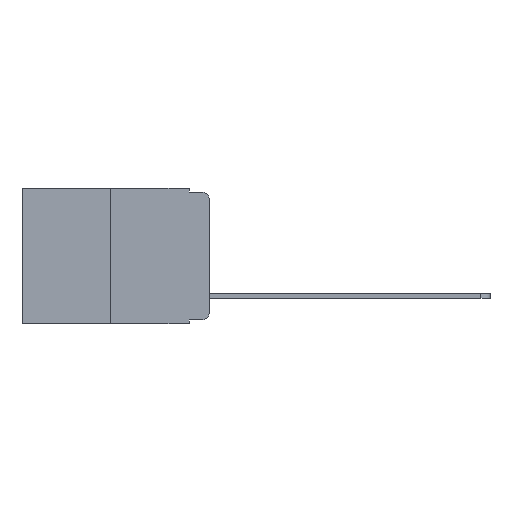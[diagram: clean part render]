
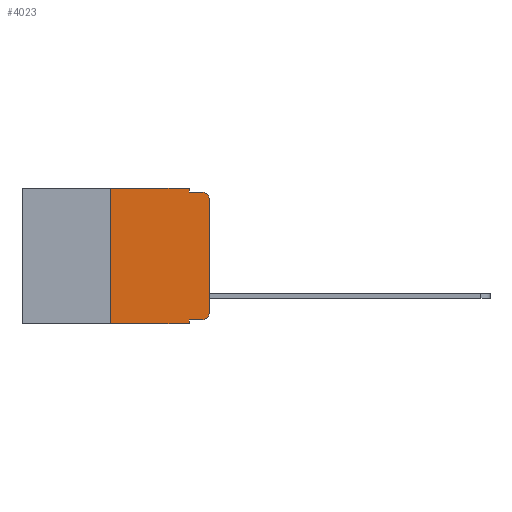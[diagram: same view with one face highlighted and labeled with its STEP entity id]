
A CAD part, left-side view. The second image highlights one B-rep face of the part: STEP entity #4023.
In plain terms, the highlighted planar face has unit normal (-1, 0, 0).
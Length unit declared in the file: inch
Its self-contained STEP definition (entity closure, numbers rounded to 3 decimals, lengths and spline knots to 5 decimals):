
#43 = PLANE ( 'NONE',  #14361 ) ;
#63 = CARTESIAN_POINT ( 'NONE',  ( 0., 0.473, 0. ) ) ;
#77 = CIRCLE ( 'NONE', #10396, 0.02 ) ;
#205 = VECTOR ( 'NONE', #4511, 39.37008 ) ;
#252 = DIRECTION ( 'NONE',  ( 1., 0., 0. ) ) ;
#527 = CARTESIAN_POINT ( 'NONE',  ( 0., 0.25, -0.343 ) ) ;
#549 = LINE ( 'NONE', #7232, #3117 ) ;
#1251 = CARTESIAN_POINT ( 'NONE',  ( 0., 0.051, -0.343 ) ) ;
#1499 = VECTOR ( 'NONE', #2564, 39.37008 ) ;
#1754 = AXIS2_PLACEMENT_3D ( 'NONE', #3244, #12026, #4750 ) ;
#2564 = DIRECTION ( 'NONE',  ( 0., -1., 0. ) ) ;
#2628 = EDGE_LOOP ( 'NONE', ( #7065, #13607, #7468, #11190, #14346, #11562, #14711, #11953, #15067, #15421 ) ) ;
#2665 = CARTESIAN_POINT ( 'NONE',  ( 0., 0.051, -0.333 ) ) ;
#3117 = VECTOR ( 'NONE', #8499, 39.37008 ) ;
#3171 = DIRECTION ( 'NONE',  ( -1., 0., 0. ) ) ;
#3209 = VECTOR ( 'NONE', #5372, 39.37008 ) ;
#3244 = CARTESIAN_POINT ( 'NONE',  ( 0., 0.02, -0.03 ) ) ;
#4023 = ADVANCED_FACE ( 'NONE', ( #10463 ), #43, .F. ) ;
#4182 = DIRECTION ( 'NONE',  ( 0., -1., 0. ) ) ;
#4190 = VECTOR ( 'NONE', #10256, 39.37008 ) ;
#4368 = DIRECTION ( 'NONE',  ( 0., 0., -1. ) ) ;
#4511 = DIRECTION ( 'NONE',  ( 0., 0., 1. ) ) ;
#4624 = VECTOR ( 'NONE', #4182, 39.37008 ) ;
#4635 = LINE ( 'NONE', #13054, #10944 ) ;
#4750 = DIRECTION ( 'NONE',  ( 0., 0., -1. ) ) ;
#5372 = DIRECTION ( 'NONE',  ( 0., 0., -1. ) ) ;
#5976 = EDGE_CURVE ( 'NONE', #7205, #10261, #10786, .T. ) ;
#6073 = CARTESIAN_POINT ( 'NONE',  ( 0., 0.02, -0.01 ) ) ;
#6177 = CARTESIAN_POINT ( 'NONE',  ( 0., 0.02, -0.333 ) ) ;
#6295 = EDGE_CURVE ( 'NONE', #7839, #15605, #77, .T. ) ;
#6835 = CIRCLE ( 'NONE', #1754, 0.02 ) ;
#6948 = LINE ( 'NONE', #7053, #205 ) ;
#7053 = CARTESIAN_POINT ( 'NONE',  ( 0., 0.25, 0. ) ) ;
#7065 = ORIENTED_EDGE ( 'NONE', *, *, #11036, .T. ) ;
#7174 = VECTOR ( 'NONE', #14970, 39.37008 ) ;
#7205 = VERTEX_POINT ( 'NONE', #10015 ) ;
#7232 = CARTESIAN_POINT ( 'NONE',  ( 0., 0.473, -0.343 ) ) ;
#7468 = ORIENTED_EDGE ( 'NONE', *, *, #5976, .F. ) ;
#7551 = LINE ( 'NONE', #2665, #4190 ) ;
#7697 = CARTESIAN_POINT ( 'NONE',  ( 0., 0., 0. ) ) ;
#7839 = VERTEX_POINT ( 'NONE', #6177 ) ;
#7983 = EDGE_CURVE ( 'NONE', #9627, #7839, #7551, .T. ) ;
#8139 = CARTESIAN_POINT ( 'NONE',  ( 0., 0., -0.313 ) ) ;
#8172 = VERTEX_POINT ( 'NONE', #11847 ) ;
#8423 = EDGE_CURVE ( 'NONE', #8839, #10991, #549, .T. ) ;
#8499 = DIRECTION ( 'NONE',  ( 0., -1., 0. ) ) ;
#8839 = VERTEX_POINT ( 'NONE', #527 ) ;
#9021 = DIRECTION ( 'NONE',  ( 0., 0., -1. ) ) ;
#9627 = VERTEX_POINT ( 'NONE', #15664 ) ;
#10015 = CARTESIAN_POINT ( 'NONE',  ( 0., 0.051, -0.01 ) ) ;
#10222 = EDGE_CURVE ( 'NONE', #13345, #10261, #6835, .T. ) ;
#10256 = DIRECTION ( 'NONE',  ( 0., -1., 0. ) ) ;
#10261 = VERTEX_POINT ( 'NONE', #6073 ) ;
#10396 = AXIS2_PLACEMENT_3D ( 'NONE', #10745, #3171, #11951 ) ;
#10463 = FACE_OUTER_BOUND ( 'NONE', #2628, .T. ) ;
#10483 = CARTESIAN_POINT ( 'NONE',  ( 0., 0.473, 0. ) ) ;
#10563 = EDGE_CURVE ( 'NONE', #8172, #14083, #14455, .T. ) ;
#10745 = CARTESIAN_POINT ( 'NONE',  ( 0., 0.02, -0.313 ) ) ;
#10786 = LINE ( 'NONE', #11365, #1499 ) ;
#10917 = LINE ( 'NONE', #7697, #7174 ) ;
#10944 = VECTOR ( 'NONE', #4368, 39.37008 ) ;
#10991 = VERTEX_POINT ( 'NONE', #1251 ) ;
#11036 = EDGE_CURVE ( 'NONE', #15605, #13345, #10917, .T. ) ;
#11190 = ORIENTED_EDGE ( 'NONE', *, *, #14502, .F. ) ;
#11331 = EDGE_CURVE ( 'NONE', #9627, #10991, #12778, .T. ) ;
#11365 = CARTESIAN_POINT ( 'NONE',  ( 0., 0.051, -0.01 ) ) ;
#11562 = ORIENTED_EDGE ( 'NONE', *, *, #12148, .F. ) ;
#11847 = CARTESIAN_POINT ( 'NONE',  ( 0., 0.25, 0. ) ) ;
#11951 = DIRECTION ( 'NONE',  ( 0., 0., -1. ) ) ;
#11953 = ORIENTED_EDGE ( 'NONE', *, *, #11331, .F. ) ;
#12026 = DIRECTION ( 'NONE',  ( -1., 0., 0. ) ) ;
#12139 = CARTESIAN_POINT ( 'NONE',  ( 0., 0., -0.03 ) ) ;
#12148 = EDGE_CURVE ( 'NONE', #8839, #8172, #6948, .T. ) ;
#12778 = LINE ( 'NONE', #13997, #3209 ) ;
#13054 = CARTESIAN_POINT ( 'NONE',  ( 0., 0.051, 0. ) ) ;
#13345 = VERTEX_POINT ( 'NONE', #12139 ) ;
#13607 = ORIENTED_EDGE ( 'NONE', *, *, #10222, .T. ) ;
#13997 = CARTESIAN_POINT ( 'NONE',  ( 0., 0.051, 0. ) ) ;
#14083 = VERTEX_POINT ( 'NONE', #14501 ) ;
#14346 = ORIENTED_EDGE ( 'NONE', *, *, #10563, .F. ) ;
#14361 = AXIS2_PLACEMENT_3D ( 'NONE', #63, #252, #9021 ) ;
#14455 = LINE ( 'NONE', #10483, #4624 ) ;
#14501 = CARTESIAN_POINT ( 'NONE',  ( 0., 0.051, 0. ) ) ;
#14502 = EDGE_CURVE ( 'NONE', #14083, #7205, #4635, .T. ) ;
#14711 = ORIENTED_EDGE ( 'NONE', *, *, #8423, .T. ) ;
#14970 = DIRECTION ( 'NONE',  ( 0., 0., 1. ) ) ;
#15067 = ORIENTED_EDGE ( 'NONE', *, *, #7983, .T. ) ;
#15421 = ORIENTED_EDGE ( 'NONE', *, *, #6295, .T. ) ;
#15605 = VERTEX_POINT ( 'NONE', #8139 ) ;
#15664 = CARTESIAN_POINT ( 'NONE',  ( 0., 0.051, -0.333 ) ) ;
